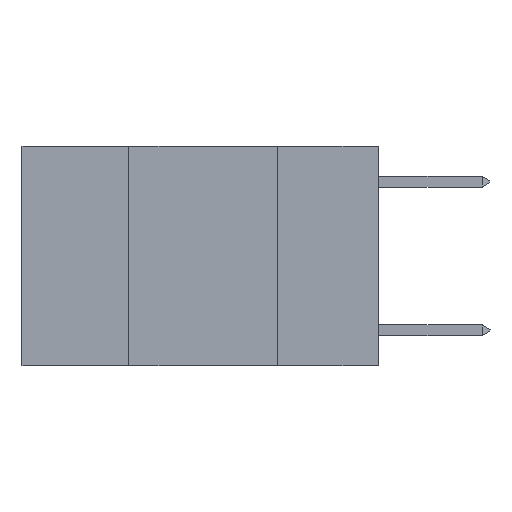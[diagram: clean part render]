
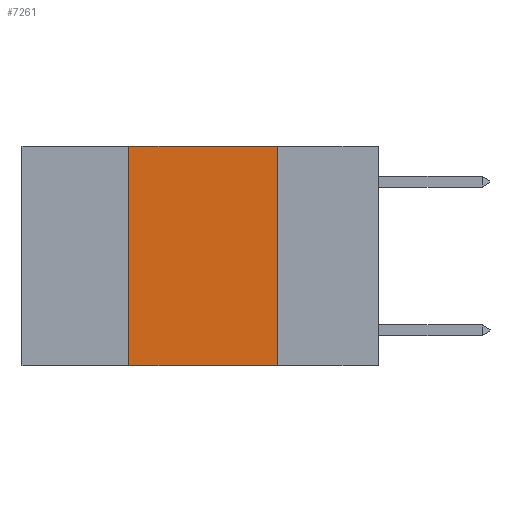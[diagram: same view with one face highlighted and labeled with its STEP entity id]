
A CAD part, left-side view. The second image highlights one B-rep face of the part: STEP entity #7261.
In plain terms, the highlighted planar face has unit normal (-1, 0, 0).
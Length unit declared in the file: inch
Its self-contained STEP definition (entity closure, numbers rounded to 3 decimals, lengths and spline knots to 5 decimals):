
#417 = CARTESIAN_POINT ( 'NONE',  ( 0., 0.6, 0. ) ) ;
#538 = CARTESIAN_POINT ( 'NONE',  ( 0., 0.42, 0. ) ) ;
#1017 = EDGE_LOOP ( 'NONE', ( #9183, #2338, #10754, #5804 ) ) ;
#1956 = VECTOR ( 'NONE', #10867, 39.37008 ) ;
#2066 = DIRECTION ( 'NONE',  ( 0., 0., -1. ) ) ;
#2338 = ORIENTED_EDGE ( 'NONE', *, *, #14590, .F. ) ;
#2603 = EDGE_CURVE ( 'NONE', #7562, #13590, #15989, .T. ) ;
#3888 = DIRECTION ( 'NONE',  ( 0., -1., 0. ) ) ;
#4437 = DIRECTION ( 'NONE',  ( 0., 0., -1. ) ) ;
#5529 = CARTESIAN_POINT ( 'NONE',  ( 0., 0.42, 0. ) ) ;
#5804 = ORIENTED_EDGE ( 'NONE', *, *, #15992, .T. ) ;
#5822 = VERTEX_POINT ( 'NONE', #15134 ) ;
#6947 = LINE ( 'NONE', #17502, #10394 ) ;
#7261 = ADVANCED_FACE ( 'NONE', ( #16221 ), #15026, .F. ) ;
#7562 = VERTEX_POINT ( 'NONE', #8438 ) ;
#8001 = CARTESIAN_POINT ( 'NONE',  ( 0., 0.17, -0.37 ) ) ;
#8438 = CARTESIAN_POINT ( 'NONE',  ( 0., 0.42, -0.37 ) ) ;
#8843 = CARTESIAN_POINT ( 'NONE',  ( 0., 0.6, 0. ) ) ;
#9183 = ORIENTED_EDGE ( 'NONE', *, *, #18648, .F. ) ;
#10394 = VECTOR ( 'NONE', #4437, 39.37008 ) ;
#10754 = ORIENTED_EDGE ( 'NONE', *, *, #2603, .F. ) ;
#10768 = DIRECTION ( 'NONE',  ( 1., 0., 0. ) ) ;
#10867 = DIRECTION ( 'NONE',  ( 0., 0., 1. ) ) ;
#11344 = VECTOR ( 'NONE', #3888, 39.37008 ) ;
#12048 = VERTEX_POINT ( 'NONE', #8001 ) ;
#12277 = AXIS2_PLACEMENT_3D ( 'NONE', #417, #10768, #2066 ) ;
#12495 = LINE ( 'NONE', #8843, #15893 ) ;
#13590 = VERTEX_POINT ( 'NONE', #5529 ) ;
#13875 = CARTESIAN_POINT ( 'NONE',  ( 0., 0.6, -0.37 ) ) ;
#14590 = EDGE_CURVE ( 'NONE', #13590, #5822, #12495, .T. ) ;
#15026 = PLANE ( 'NONE',  #12277 ) ;
#15134 = CARTESIAN_POINT ( 'NONE',  ( 0., 0.17, 0. ) ) ;
#15893 = VECTOR ( 'NONE', #18782, 39.37008 ) ;
#15989 = LINE ( 'NONE', #538, #1956 ) ;
#15992 = EDGE_CURVE ( 'NONE', #7562, #12048, #16068, .T. ) ;
#16068 = LINE ( 'NONE', #13875, #11344 ) ;
#16221 = FACE_OUTER_BOUND ( 'NONE', #1017, .T. ) ;
#17502 = CARTESIAN_POINT ( 'NONE',  ( 0., 0.17, 0. ) ) ;
#18648 = EDGE_CURVE ( 'NONE', #5822, #12048, #6947, .T. ) ;
#18782 = DIRECTION ( 'NONE',  ( 0., -1., 0. ) ) ;
